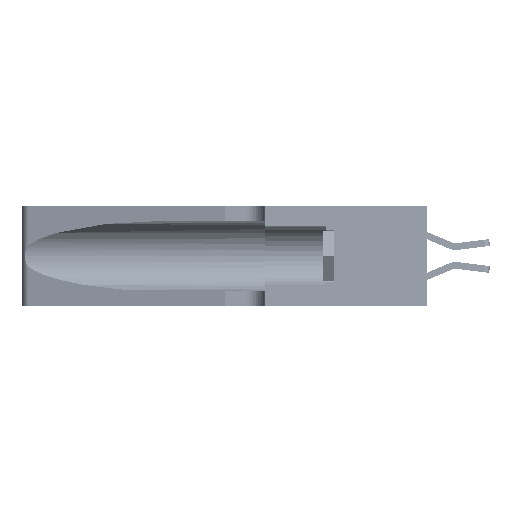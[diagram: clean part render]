
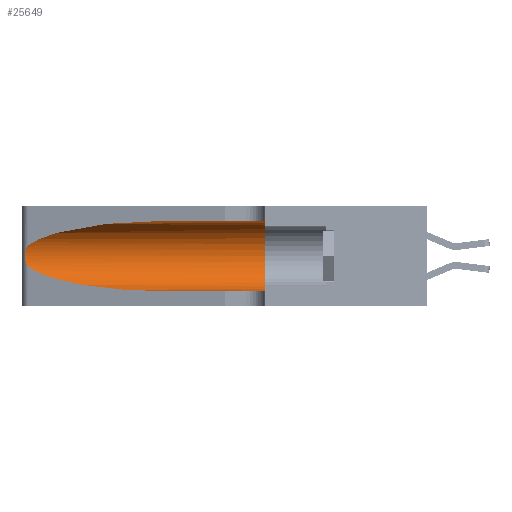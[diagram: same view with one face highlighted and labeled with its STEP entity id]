
A CAD part, left-side view. The second image highlights one B-rep face of the part: STEP entity #25649.
In plain terms, the highlighted cylindrical face has radius 3.308 mm (diameter 6.617 mm), a partial arc.
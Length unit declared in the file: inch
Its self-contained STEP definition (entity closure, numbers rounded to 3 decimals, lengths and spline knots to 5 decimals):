
#326 = ORIENTED_EDGE ( 'NONE', *, *, #33278, .T. ) ;
#853 = CARTESIAN_POINT ( 'NONE',  ( 0.26075, 1.23896, 0.19203 ) ) ;
#1036 = ORIENTED_EDGE ( 'NONE', *, *, #28651, .T. ) ;
#1636 = CARTESIAN_POINT ( 'NONE',  ( 0.1305, 0.35, 0.185 ) ) ;
#2886 = VERTEX_POINT ( 'NONE', #6773 ) ;
#3634 =( BOUNDED_CURVE ( )  B_SPLINE_CURVE ( 3, ( #15326, #32017, #11350, #40351 ),
 .UNSPECIFIED., .F., .F. ) 
 B_SPLINE_CURVE_WITH_KNOTS ( ( 4, 4 ),
 ( 3.44316, 4.71239 ),
 .UNSPECIFIED. ) 
 CURVE ( )  GEOMETRIC_REPRESENTATION_ITEM ( )  RATIONAL_B_SPLINE_CURVE ( ( 1., 0.87, 0.87, 1. ) ) 
 REPRESENTATION_ITEM ( '' )  );
#4723 = FACE_OUTER_BOUND ( 'NONE', #7754, .T. ) ;
#5021 = CARTESIAN_POINT ( 'NONE',  ( 0.26017, 1.23833, 0.17102 ) ) ;
#5165 = EDGE_CURVE ( 'NONE', #52313, #14674, #50470, .T. ) ;
#5598 = CARTESIAN_POINT ( 'NONE',  ( 0.1305, 0.72297, 0.31525 ) ) ;
#5837 = DIRECTION ( 'NONE',  ( 0., 0., 1. ) ) ;
#6773 = CARTESIAN_POINT ( 'NONE',  ( 0.25487, 1.22718, 0.14631 ) ) ;
#6788 = DIRECTION ( 'NONE',  ( 0., 0., -1. ) ) ;
#7216 = ORIENTED_EDGE ( 'NONE', *, *, #5165, .T. ) ;
#7754 = EDGE_LOOP ( 'NONE', ( #49975, #1036, #326, #7216, #48363, #10795 ) ) ;
#7960 = CARTESIAN_POINT ( 'NONE',  ( 0.25487, 1.22718, 0.22369 ) ) ;
#8747 = CARTESIAN_POINT ( 'NONE',  ( 0.1305, 1.61858, 0.05475 ) ) ;
#8844 = CARTESIAN_POINT ( 'NONE',  ( 0.25487, 1.22718, 0.22369 ) ) ;
#9211 = CARTESIAN_POINT ( 'NONE',  ( 0.25789, 1.23486, 0.15765 ) ) ;
#9430 = CARTESIAN_POINT ( 'NONE',  ( 0.1305, 0.72297, 0.05475 ) ) ;
#9496 = EDGE_CURVE ( 'NONE', #32609, #14674, #15201, .T. ) ;
#10795 = ORIENTED_EDGE ( 'NONE', *, *, #37821, .F. ) ;
#11043 = VERTEX_POINT ( 'NONE', #35918 ) ;
#11350 = CARTESIAN_POINT ( 'NONE',  ( 0.18966, 0.96281, 0.05475 ) ) ;
#13132 = CYLINDRICAL_SURFACE ( 'NONE', #14472, 0.13025 ) ;
#13162 = CARTESIAN_POINT ( 'NONE',  ( 0.25555, 1.22994, 0.2215 ) ) ;
#13336 = CARTESIAN_POINT ( 'NONE',  ( 0.25555, 1.22993, 0.14849 ) ) ;
#14472 = AXIS2_PLACEMENT_3D ( 'NONE', #48071, #52223, #6788 ) ;
#14674 = VERTEX_POINT ( 'NONE', #26296 ) ;
#15201 = CIRCLE ( 'NONE', #30698, 0.13025 ) ;
#15325 = EDGE_CURVE ( 'NONE', #11043, #47858, #34203, .T. ) ;
#15326 = CARTESIAN_POINT ( 'NONE',  ( 0.25487, 1.22718, 0.14631 ) ) ;
#15690 = CARTESIAN_POINT ( 'NONE',  ( 0.1305, 1.61858, 0.31525 ) ) ;
#17049 = VECTOR ( 'NONE', #40529, 39.37008 ) ;
#18075 = CARTESIAN_POINT ( 'NONE',  ( 0.25487, 1.22718, 0.22369 ) ) ;
#18657 = VECTOR ( 'NONE', #33549, 39.37008 ) ;
#21502 = CARTESIAN_POINT ( 'NONE',  ( 0.25787, 1.23484, 0.2124 ) ) ;
#25649 = ADVANCED_FACE ( 'NONE', ( #4723 ), #13132, .F. ) ;
#25672 = CARTESIAN_POINT ( 'NONE',  ( 0.26018, 1.23835, 0.19895 ) ) ;
#26296 = CARTESIAN_POINT ( 'NONE',  ( 0.1305, 0.35, 0.05475 ) ) ;
#28556 = B_SPLINE_CURVE_WITH_KNOTS ( 'NONE', 3,
 ( #8844, #13162, #46334, #21502, #50512, #25672, #853, #29832, #5021, #34005, #9211, #38165, #13336, #42338 ),
 .UNSPECIFIED., .F., .F.,
 ( 4, 2, 2, 2, 2, 2, 4 ),
 ( 0., 0.00027, 0.00053, 0.00107, 0.0016, 0.00187, 0.00214 ),
 .UNSPECIFIED. ) ;
#28651 = EDGE_CURVE ( 'NONE', #47858, #2886, #28556, .T. ) ;
#29353 = LINE ( 'NONE', #15690, #17049 ) ;
#29832 = CARTESIAN_POINT ( 'NONE',  ( 0.26075, 1.23896, 0.178 ) ) ;
#30398 = CARTESIAN_POINT ( 'NONE',  ( 0.18966, 0.96281, 0.31525 ) ) ;
#30645 = DIRECTION ( 'NONE',  ( 0., 1., 0. ) ) ;
#30698 = AXIS2_PLACEMENT_3D ( 'NONE', #1636, #30645, #5837 ) ;
#32017 = CARTESIAN_POINT ( 'NONE',  ( 0.2373, 1.15595, 0.08982 ) ) ;
#32609 = VERTEX_POINT ( 'NONE', #37112 ) ;
#33278 = EDGE_CURVE ( 'NONE', #2886, #52313, #3634, .T. ) ;
#33549 = DIRECTION ( 'NONE',  ( 0., -1., 0. ) ) ;
#34005 = CARTESIAN_POINT ( 'NONE',  ( 0.25856, 1.23593, 0.16098 ) ) ;
#34203 =( BOUNDED_CURVE ( )  B_SPLINE_CURVE ( 3, ( #5598, #30398, #42903, #18075 ),
 .UNSPECIFIED., .F., .T. ) 
 B_SPLINE_CURVE_WITH_KNOTS ( ( 4, 4 ),
 ( 1.5708, 2.84003 ),
 .UNSPECIFIED. ) 
 CURVE ( )  GEOMETRIC_REPRESENTATION_ITEM ( )  RATIONAL_B_SPLINE_CURVE ( ( 1., 0.87, 0.87, 1. ) ) 
 REPRESENTATION_ITEM ( '' )  );
#35918 = CARTESIAN_POINT ( 'NONE',  ( 0.1305, 0.72297, 0.31525 ) ) ;
#37112 = CARTESIAN_POINT ( 'NONE',  ( 0.1305, 0.35, 0.31525 ) ) ;
#37821 = EDGE_CURVE ( 'NONE', #11043, #32609, #29353, .T. ) ;
#38165 = CARTESIAN_POINT ( 'NONE',  ( 0.25639, 1.23186, 0.15144 ) ) ;
#40351 = CARTESIAN_POINT ( 'NONE',  ( 0.1305, 0.72297, 0.05475 ) ) ;
#40529 = DIRECTION ( 'NONE',  ( 0., -1., 0. ) ) ;
#42338 = CARTESIAN_POINT ( 'NONE',  ( 0.25487, 1.22718, 0.14631 ) ) ;
#42903 = CARTESIAN_POINT ( 'NONE',  ( 0.2373, 1.15595, 0.28018 ) ) ;
#46334 = CARTESIAN_POINT ( 'NONE',  ( 0.25639, 1.23184, 0.21858 ) ) ;
#47858 = VERTEX_POINT ( 'NONE', #7960 ) ;
#48071 = CARTESIAN_POINT ( 'NONE',  ( 0.1305, 1.61858, 0.185 ) ) ;
#48363 = ORIENTED_EDGE ( 'NONE', *, *, #9496, .F. ) ;
#49975 = ORIENTED_EDGE ( 'NONE', *, *, #15325, .T. ) ;
#50470 = LINE ( 'NONE', #8747, #18657 ) ;
#50512 = CARTESIAN_POINT ( 'NONE',  ( 0.25854, 1.2359, 0.20912 ) ) ;
#52223 = DIRECTION ( 'NONE',  ( 0., -1., 0. ) ) ;
#52313 = VERTEX_POINT ( 'NONE', #9430 ) ;
